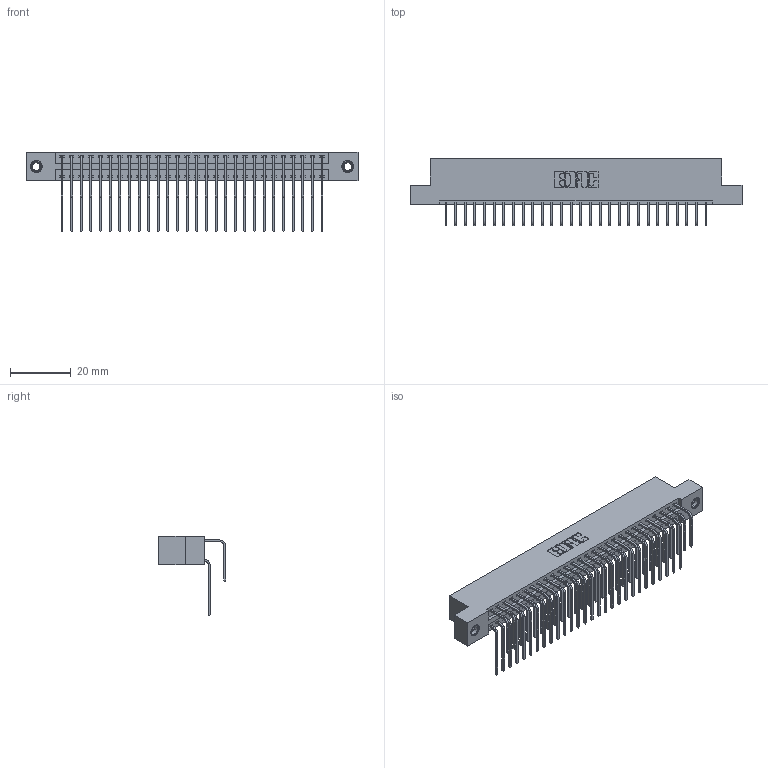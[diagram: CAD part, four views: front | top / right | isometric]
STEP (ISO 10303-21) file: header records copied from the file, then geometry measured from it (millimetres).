
FILE_DESCRIPTION (( 'STEP AP203' ), '1' );
FILE_NAME ('346-056-558-207.STEP', '2022-05-21T06:41:06', ( '' ), ( '' ), 'SwSTEP 2.0', 'SolidWorks 2020', '' );
FILE_SCHEMA (( 'CONFIG_CONTROL_DESIGN' ));
Length unit declared in the file: inch
Products named in the file (5): 346 Part_Flush Mounting Lugs - 0.156 Dia-TI; 345-250-001_345-250-005-103; 346-056-558-207; 345-292-001_558 559 Tail - 1; 345-292-001_558 Tail - 2
Assembly tree (59 placements, depth 2):
  346-056-558-207
    346 Part_Flush Mounting Lugs - 0.156 Dia-TI
    345-292-001_558 559 Tail - 1  x28
    345-292-001_558 Tail - 2  x28
    345-250-001_345-250-005-103  x2
Bounding box: 109.47 x 22.16 x 26.16 mm (x, y, z)
Volume: 10875.9 mm3; surface area: 16313.1 mm2
Topology: 59 solids, 59 shells, 3206 faces, 9481 edges, 6238 vertices
Faces by surface type: plane 2180, cylinder 1010, cone 12, torus 4
Entity records: 23128 total; most frequent: CARTESIAN_POINT 3866, ORIENTED_EDGE 3742, DIRECTION 3457, EDGE_CURVE 1871, LINE 1567, VECTOR 1567, VERTEX_POINT 1240, AXIS2_PLACEMENT_3D 945
